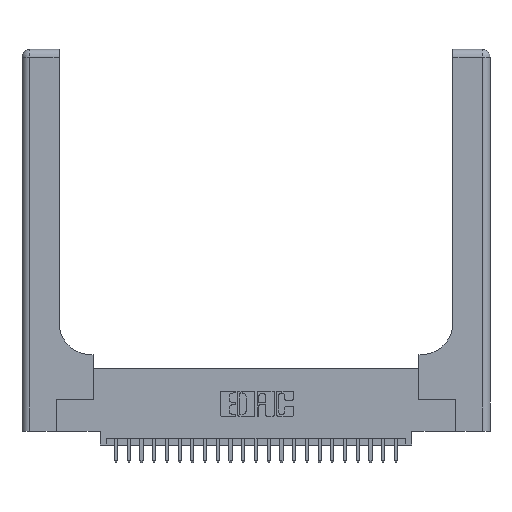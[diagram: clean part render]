
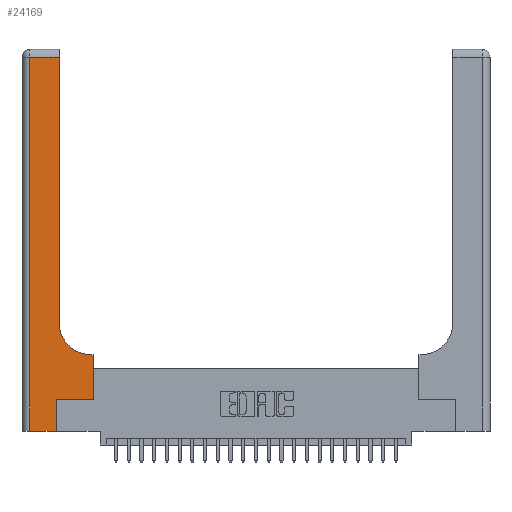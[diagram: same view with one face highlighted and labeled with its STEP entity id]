
A CAD part, top view. The second image highlights one B-rep face of the part: STEP entity #24169.
In plain terms, the highlighted planar face has unit normal (0, 0, 1).
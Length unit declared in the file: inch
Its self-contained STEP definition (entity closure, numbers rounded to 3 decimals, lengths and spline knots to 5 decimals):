
#387 = EDGE_CURVE ( 'NONE', #18351, #3635, #757, .T. ) ;
#496 = CARTESIAN_POINT ( 'NONE',  ( 0., 2.94, 0.37 ) ) ;
#499 = FACE_OUTER_BOUND ( 'NONE', #9811, .T. ) ;
#623 = ORIENTED_EDGE ( 'NONE', *, *, #25782, .T. ) ;
#757 = LINE ( 'NONE', #7944, #14590 ) ;
#803 = VERTEX_POINT ( 'NONE', #23176 ) ;
#1426 = CARTESIAN_POINT ( 'NONE',  ( 0., 0., 0.37 ) ) ;
#1659 = CARTESIAN_POINT ( 'NONE',  ( 0.269, 0.25, 0.37 ) ) ;
#1750 = ORIENTED_EDGE ( 'NONE', *, *, #14330, .T. ) ;
#2311 = VECTOR ( 'NONE', #15702, 39.37008 ) ;
#3635 = VERTEX_POINT ( 'NONE', #20393 ) ;
#3747 = CARTESIAN_POINT ( 'NONE',  ( 0.269, 0., 0.37 ) ) ;
#3836 = LINE ( 'NONE', #19901, #25158 ) ;
#4232 = LINE ( 'NONE', #1659, #2311 ) ;
#4479 = LINE ( 'NONE', #3747, #22357 ) ;
#4521 = CARTESIAN_POINT ( 'NONE',  ( 0., 3., 0.37 ) ) ;
#5591 = VERTEX_POINT ( 'NONE', #14354 ) ;
#6738 = LINE ( 'NONE', #9781, #22737 ) ;
#7309 = EDGE_CURVE ( 'NONE', #5591, #18351, #21998, .T. ) ;
#7495 = DIRECTION ( 'NONE',  ( 1., 0., 0. ) ) ;
#7940 = AXIS2_PLACEMENT_3D ( 'NONE', #8412, #12410, #22605 ) ;
#7944 = CARTESIAN_POINT ( 'NONE',  ( 0.2915, 3., 0.37 ) ) ;
#8352 = CARTESIAN_POINT ( 'NONE',  ( 0.269, 0.25, 0.37 ) ) ;
#8412 = CARTESIAN_POINT ( 'NONE',  ( 0.5415, 0.85, 0.37 ) ) ;
#9781 = CARTESIAN_POINT ( 'NONE',  ( 0.2915, 0.6, 0.37 ) ) ;
#9811 = EDGE_LOOP ( 'NONE', ( #10992, #20910, #1750, #12198, #623, #18388, #20546, #12542, #20119 ) ) ;
#10293 = DIRECTION ( 'NONE',  ( 0., 1., 0. ) ) ;
#10850 = VECTOR ( 'NONE', #10293, 39.37008 ) ;
#10992 = ORIENTED_EDGE ( 'NONE', *, *, #387, .T. ) ;
#12112 = DIRECTION ( 'NONE',  ( -1., 0., 0. ) ) ;
#12198 = ORIENTED_EDGE ( 'NONE', *, *, #18884, .T. ) ;
#12410 = DIRECTION ( 'NONE',  ( 0., 0., -1. ) ) ;
#12542 = ORIENTED_EDGE ( 'NONE', *, *, #24582, .T. ) ;
#12642 = VERTEX_POINT ( 'NONE', #22885 ) ;
#12725 = DIRECTION ( 'NONE',  ( 0., 0., -1. ) ) ;
#13765 = CARTESIAN_POINT ( 'NONE',  ( 0.269, 0., 0.37 ) ) ;
#13836 = EDGE_CURVE ( 'NONE', #3635, #21690, #18600, .T. ) ;
#14160 = DIRECTION ( 'NONE',  ( 0., 1., 0. ) ) ;
#14330 = EDGE_CURVE ( 'NONE', #21690, #803, #3836, .T. ) ;
#14354 = CARTESIAN_POINT ( 'NONE',  ( 0.5415, 0.6, 0.37 ) ) ;
#14590 = VECTOR ( 'NONE', #14160, 39.37008 ) ;
#14649 = AXIS2_PLACEMENT_3D ( 'NONE', #4521, #12725, #22482 ) ;
#14657 = CARTESIAN_POINT ( 'NONE',  ( 0.5585, 0.25, 0.37 ) ) ;
#15089 = LINE ( 'NONE', #1426, #21682 ) ;
#15702 = DIRECTION ( 'NONE',  ( 1., 0., 0. ) ) ;
#16102 = CARTESIAN_POINT ( 'NONE',  ( 0.5585, 0.25, 0.37 ) ) ;
#16357 = CARTESIAN_POINT ( 'NONE',  ( 0.06, 2.94, 0.37 ) ) ;
#16494 = LINE ( 'NONE', #16102, #10850 ) ;
#16719 = PLANE ( 'NONE',  #14649 ) ;
#17639 = VERTEX_POINT ( 'NONE', #8352 ) ;
#17954 = VERTEX_POINT ( 'NONE', #13765 ) ;
#18351 = VERTEX_POINT ( 'NONE', #19603 ) ;
#18388 = ORIENTED_EDGE ( 'NONE', *, *, #25109, .T. ) ;
#18600 = LINE ( 'NONE', #496, #25511 ) ;
#18884 = EDGE_CURVE ( 'NONE', #803, #17954, #15089, .T. ) ;
#19343 = VERTEX_POINT ( 'NONE', #14657 ) ;
#19603 = CARTESIAN_POINT ( 'NONE',  ( 0.2915, 0.85, 0.37 ) ) ;
#19901 = CARTESIAN_POINT ( 'NONE',  ( 0.06, 3., 0.37 ) ) ;
#20119 = ORIENTED_EDGE ( 'NONE', *, *, #7309, .T. ) ;
#20393 = CARTESIAN_POINT ( 'NONE',  ( 0.2915, 2.94, 0.37 ) ) ;
#20546 = ORIENTED_EDGE ( 'NONE', *, *, #21669, .T. ) ;
#20910 = ORIENTED_EDGE ( 'NONE', *, *, #13836, .T. ) ;
#21669 = EDGE_CURVE ( 'NONE', #19343, #12642, #16494, .T. ) ;
#21682 = VECTOR ( 'NONE', #7495, 39.37008 ) ;
#21690 = VERTEX_POINT ( 'NONE', #16357 ) ;
#21998 = CIRCLE ( 'NONE', #7940, 0.25 ) ;
#22357 = VECTOR ( 'NONE', #23685, 39.37008 ) ;
#22482 = DIRECTION ( 'NONE',  ( -1., 0., 0. ) ) ;
#22495 = DIRECTION ( 'NONE',  ( -1., 0., 0. ) ) ;
#22605 = DIRECTION ( 'NONE',  ( 1., 0., 0. ) ) ;
#22737 = VECTOR ( 'NONE', #12112, 39.37008 ) ;
#22885 = CARTESIAN_POINT ( 'NONE',  ( 0.5585, 0.6, 0.37 ) ) ;
#23176 = CARTESIAN_POINT ( 'NONE',  ( 0.06, 0., 0.37 ) ) ;
#23685 = DIRECTION ( 'NONE',  ( 0., 1., 0. ) ) ;
#24169 = ADVANCED_FACE ( 'NONE', ( #499 ), #16719, .F. ) ;
#24582 = EDGE_CURVE ( 'NONE', #12642, #5591, #6738, .T. ) ;
#25109 = EDGE_CURVE ( 'NONE', #17639, #19343, #4232, .T. ) ;
#25158 = VECTOR ( 'NONE', #25859, 39.37008 ) ;
#25511 = VECTOR ( 'NONE', #22495, 39.37008 ) ;
#25782 = EDGE_CURVE ( 'NONE', #17954, #17639, #4479, .T. ) ;
#25859 = DIRECTION ( 'NONE',  ( 0., -1., 0. ) ) ;
